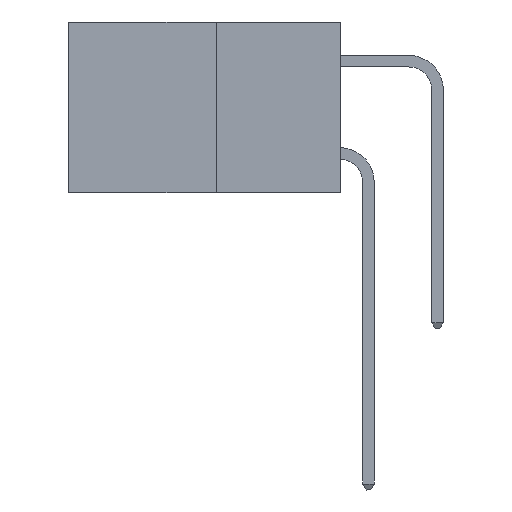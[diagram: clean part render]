
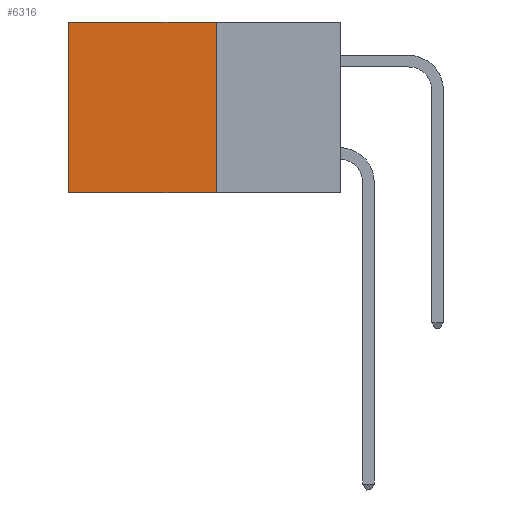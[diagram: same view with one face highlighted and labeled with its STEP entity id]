
A CAD part, left-side view. The second image highlights one B-rep face of the part: STEP entity #6316.
In plain terms, the highlighted planar face has unit normal (-1, 0, 0).
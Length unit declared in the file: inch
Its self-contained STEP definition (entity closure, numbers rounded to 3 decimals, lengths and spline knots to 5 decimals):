
#202 = VERTEX_POINT ( 'NONE', #8382 ) ;
#501 = VERTEX_POINT ( 'NONE', #7407 ) ;
#606 = EDGE_CURVE ( 'NONE', #202, #4557, #1233, .T. ) ;
#772 = EDGE_CURVE ( 'NONE', #4401, #202, #3436, .T. ) ;
#845 = EDGE_CURVE ( 'NONE', #4401, #501, #8377, .T. ) ;
#918 = VECTOR ( 'NONE', #6600, 39.37008 ) ;
#1116 = ORIENTED_EDGE ( 'NONE', *, *, #606, .T. ) ;
#1233 = LINE ( 'NONE', #7681, #918 ) ;
#1720 = CARTESIAN_POINT ( 'NONE',  ( 0.277, 0.27, 0. ) ) ;
#1786 = EDGE_LOOP ( 'NONE', ( #1116, #5865, #7845, #9766 ) ) ;
#1857 = DIRECTION ( 'NONE',  ( 0., 1., 0. ) ) ;
#1937 = DIRECTION ( 'NONE',  ( 0., 0., -1. ) ) ;
#2388 = CARTESIAN_POINT ( 'NONE',  ( 0.277, 0.27, -0.37 ) ) ;
#2618 = VECTOR ( 'NONE', #10268, 39.37008 ) ;
#3229 = LINE ( 'NONE', #9590, #2618 ) ;
#3436 = LINE ( 'NONE', #1720, #7338 ) ;
#4183 = EDGE_CURVE ( 'NONE', #501, #4557, #3229, .T. ) ;
#4401 = VERTEX_POINT ( 'NONE', #7634 ) ;
#4557 = VERTEX_POINT ( 'NONE', #8515 ) ;
#5865 = ORIENTED_EDGE ( 'NONE', *, *, #4183, .F. ) ;
#6216 = CARTESIAN_POINT ( 'NONE',  ( 0.277, 0.27, -0.37 ) ) ;
#6316 = ADVANCED_FACE ( 'NONE', ( #8993 ), #8427, .F. ) ;
#6408 = VECTOR ( 'NONE', #8770, 39.37008 ) ;
#6600 = DIRECTION ( 'NONE',  ( 0., 0., -1. ) ) ;
#6986 = DIRECTION ( 'NONE',  ( 1., 0., 0. ) ) ;
#7338 = VECTOR ( 'NONE', #1857, 39.37008 ) ;
#7407 = CARTESIAN_POINT ( 'NONE',  ( 0.277, 0.27, -0.37 ) ) ;
#7634 = CARTESIAN_POINT ( 'NONE',  ( 0.277, 0.27, 0. ) ) ;
#7681 = CARTESIAN_POINT ( 'NONE',  ( 0.277, 0.59, -0.37 ) ) ;
#7845 = ORIENTED_EDGE ( 'NONE', *, *, #845, .F. ) ;
#8377 = LINE ( 'NONE', #2388, #6408 ) ;
#8382 = CARTESIAN_POINT ( 'NONE',  ( 0.277, 0.59, 0. ) ) ;
#8427 = PLANE ( 'NONE',  #9634 ) ;
#8515 = CARTESIAN_POINT ( 'NONE',  ( 0.277, 0.59, -0.37 ) ) ;
#8770 = DIRECTION ( 'NONE',  ( 0., 0., -1. ) ) ;
#8993 = FACE_OUTER_BOUND ( 'NONE', #1786, .T. ) ;
#9590 = CARTESIAN_POINT ( 'NONE',  ( 0.277, 0.27, -0.37 ) ) ;
#9634 = AXIS2_PLACEMENT_3D ( 'NONE', #6216, #6986, #1937 ) ;
#9766 = ORIENTED_EDGE ( 'NONE', *, *, #772, .T. ) ;
#10268 = DIRECTION ( 'NONE',  ( 0., 1., 0. ) ) ;
